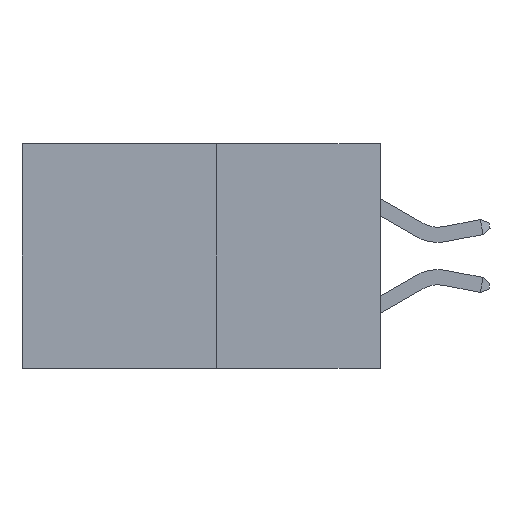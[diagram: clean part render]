
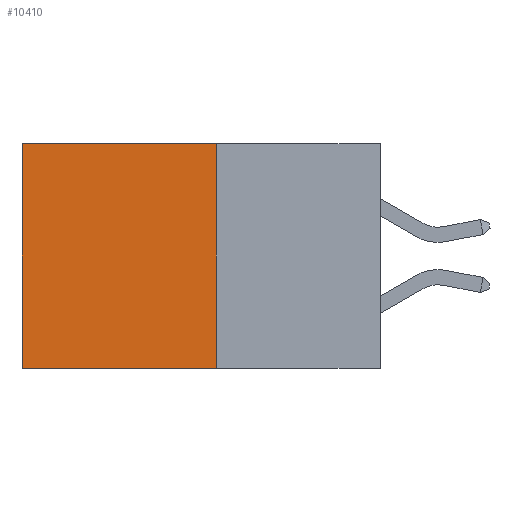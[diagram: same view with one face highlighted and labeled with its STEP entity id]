
A CAD part, left-side view. The second image highlights one B-rep face of the part: STEP entity #10410.
In plain terms, the highlighted planar face has unit normal (-1, 0, 0).
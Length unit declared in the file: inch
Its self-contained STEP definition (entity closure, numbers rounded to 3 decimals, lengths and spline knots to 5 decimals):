
#383 = FACE_OUTER_BOUND ( 'NONE', #2631, .T. ) ;
#456 = EDGE_CURVE ( 'NONE', #10689, #4321, #7673, .T. ) ;
#619 = EDGE_CURVE ( 'NONE', #5025, #4321, #5884, .T. ) ;
#1222 = VECTOR ( 'NONE', #7357, 39.37008 ) ;
#1255 = EDGE_CURVE ( 'NONE', #2526, #5025, #8312, .T. ) ;
#1973 = CARTESIAN_POINT ( 'NONE',  ( 0.277, 0.27, -0.37 ) ) ;
#2112 = CARTESIAN_POINT ( 'NONE',  ( 0.277, 0.59, -0.37 ) ) ;
#2275 = ORIENTED_EDGE ( 'NONE', *, *, #619, .T. ) ;
#2526 = VERTEX_POINT ( 'NONE', #10580 ) ;
#2585 = CARTESIAN_POINT ( 'NONE',  ( 0.277, 0.59, -0.37 ) ) ;
#2631 = EDGE_LOOP ( 'NONE', ( #2275, #5132, #8443, #9928 ) ) ;
#3345 = CARTESIAN_POINT ( 'NONE',  ( 0.277, 0.59, 0. ) ) ;
#3554 = AXIS2_PLACEMENT_3D ( 'NONE', #1973, #11762, #6556 ) ;
#4321 = VERTEX_POINT ( 'NONE', #2585 ) ;
#4968 = DIRECTION ( 'NONE',  ( 0., 1., 0. ) ) ;
#5025 = VERTEX_POINT ( 'NONE', #3345 ) ;
#5132 = ORIENTED_EDGE ( 'NONE', *, *, #456, .F. ) ;
#5202 = VECTOR ( 'NONE', #7698, 39.37008 ) ;
#5320 = VECTOR ( 'NONE', #10903, 39.37008 ) ;
#5582 = EDGE_CURVE ( 'NONE', #2526, #10689, #5615, .T. ) ;
#5615 = LINE ( 'NONE', #11327, #5320 ) ;
#5884 = LINE ( 'NONE', #2112, #1222 ) ;
#6556 = DIRECTION ( 'NONE',  ( 0., 0., -1. ) ) ;
#7357 = DIRECTION ( 'NONE',  ( 0., 0., -1. ) ) ;
#7673 = LINE ( 'NONE', #11417, #5202 ) ;
#7698 = DIRECTION ( 'NONE',  ( 0., 1., 0. ) ) ;
#7800 = CARTESIAN_POINT ( 'NONE',  ( 0.277, 0.27, -0.37 ) ) ;
#8026 = VECTOR ( 'NONE', #4968, 39.37008 ) ;
#8312 = LINE ( 'NONE', #10761, #8026 ) ;
#8443 = ORIENTED_EDGE ( 'NONE', *, *, #5582, .F. ) ;
#9928 = ORIENTED_EDGE ( 'NONE', *, *, #1255, .T. ) ;
#10071 = PLANE ( 'NONE',  #3554 ) ;
#10410 = ADVANCED_FACE ( 'NONE', ( #383 ), #10071, .F. ) ;
#10580 = CARTESIAN_POINT ( 'NONE',  ( 0.277, 0.27, 0. ) ) ;
#10689 = VERTEX_POINT ( 'NONE', #7800 ) ;
#10761 = CARTESIAN_POINT ( 'NONE',  ( 0.277, 0.27, 0. ) ) ;
#10903 = DIRECTION ( 'NONE',  ( 0., 0., -1. ) ) ;
#11327 = CARTESIAN_POINT ( 'NONE',  ( 0.277, 0.27, -0.37 ) ) ;
#11417 = CARTESIAN_POINT ( 'NONE',  ( 0.277, 0.27, -0.37 ) ) ;
#11762 = DIRECTION ( 'NONE',  ( 1., 0., 0. ) ) ;
